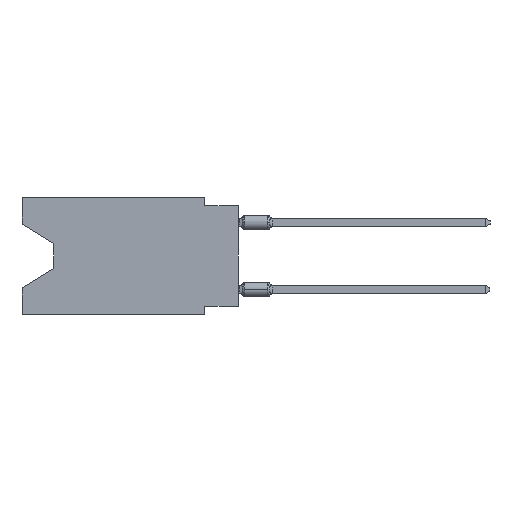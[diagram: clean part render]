
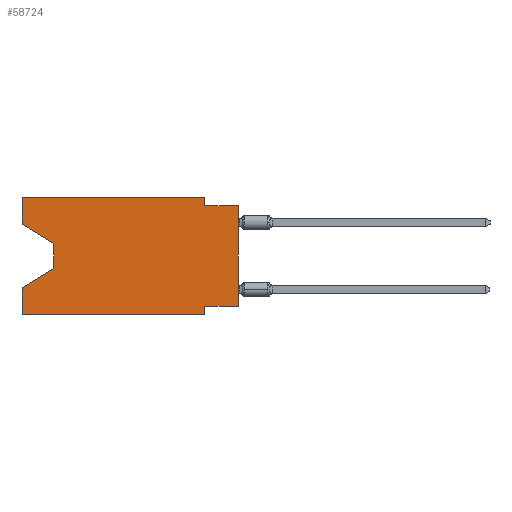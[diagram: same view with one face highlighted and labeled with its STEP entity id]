
A CAD part, left-side view. The second image highlights one B-rep face of the part: STEP entity #58724.
In plain terms, the highlighted planar face has unit normal (-1, 0, 0).
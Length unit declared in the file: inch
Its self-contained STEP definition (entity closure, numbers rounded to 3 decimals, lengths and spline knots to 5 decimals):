
#293 = VERTEX_POINT ( 'NONE', #399 ) ;
#399 = CARTESIAN_POINT ( 'NONE',  ( 0., 0.645, -0.35 ) ) ;
#412 = CARTESIAN_POINT ( 'NONE',  ( 0., 0., -0.325 ) ) ;
#1284 = VERTEX_POINT ( 'NONE', #28639 ) ;
#1549 = DIRECTION ( 'NONE',  ( 0., 0., -1. ) ) ;
#2356 = VECTOR ( 'NONE', #36975, 39.37008 ) ;
#4718 = ORIENTED_EDGE ( 'NONE', *, *, #58949, .F. ) ;
#4814 = VERTEX_POINT ( 'NONE', #9503 ) ;
#4859 = ORIENTED_EDGE ( 'NONE', *, *, #10549, .F. ) ;
#5042 = CARTESIAN_POINT ( 'NONE',  ( 0., 0.1, 0. ) ) ;
#6715 = CARTESIAN_POINT ( 'NONE',  ( 0., 0.645, -0.08025 ) ) ;
#7134 = EDGE_CURVE ( 'NONE', #57390, #23682, #11436, .T. ) ;
#7167 = DIRECTION ( 'NONE',  ( 0., -1., 0. ) ) ;
#7560 = EDGE_CURVE ( 'NONE', #19858, #56398, #16122, .T. ) ;
#7784 = ORIENTED_EDGE ( 'NONE', *, *, #7134, .T. ) ;
#8403 = CARTESIAN_POINT ( 'NONE',  ( 0., 0.645, 0. ) ) ;
#8684 = ORIENTED_EDGE ( 'NONE', *, *, #8702, .T. ) ;
#8702 = EDGE_CURVE ( 'NONE', #293, #1284, #29754, .T. ) ;
#9482 = CARTESIAN_POINT ( 'NONE',  ( 0., 0.645, 0. ) ) ;
#9503 = CARTESIAN_POINT ( 'NONE',  ( 0., 0.645, 0. ) ) ;
#9857 = VERTEX_POINT ( 'NONE', #5042 ) ;
#9894 = EDGE_CURVE ( 'NONE', #4814, #9857, #15497, .T. ) ;
#10064 = VECTOR ( 'NONE', #11071, 39.37008 ) ;
#10549 = EDGE_CURVE ( 'NONE', #57390, #4814, #12846, .T. ) ;
#10797 = CARTESIAN_POINT ( 'NONE',  ( 0., 0.55, -0.212 ) ) ;
#11071 = DIRECTION ( 'NONE',  ( 0., -1., 0. ) ) ;
#11100 = VERTEX_POINT ( 'NONE', #32286 ) ;
#11254 = ORIENTED_EDGE ( 'NONE', *, *, #7560, .T. ) ;
#11359 = DIRECTION ( 'NONE',  ( 0., 0., 1. ) ) ;
#11436 = LINE ( 'NONE', #6715, #28349 ) ;
#11443 = DIRECTION ( 'NONE',  ( 0., 0., -1. ) ) ;
#12846 = LINE ( 'NONE', #8403, #32536 ) ;
#15497 = LINE ( 'NONE', #9482, #42504 ) ;
#15634 = ORIENTED_EDGE ( 'NONE', *, *, #29944, .F. ) ;
#15951 = CARTESIAN_POINT ( 'NONE',  ( 0., 0., -0.025 ) ) ;
#16122 = LINE ( 'NONE', #30372, #46452 ) ;
#16690 = DIRECTION ( 'NONE',  ( 1., 0., 0. ) ) ;
#17109 = DIRECTION ( 'NONE',  ( 0., -0.855, -0.519 ) ) ;
#17300 = FACE_OUTER_BOUND ( 'NONE', #20377, .T. ) ;
#17316 = DIRECTION ( 'NONE',  ( 0., 1., 0. ) ) ;
#17318 = LINE ( 'NONE', #33125, #2356 ) ;
#18092 = ORIENTED_EDGE ( 'NONE', *, *, #35099, .F. ) ;
#18210 = LINE ( 'NONE', #47348, #30458 ) ;
#19685 = LINE ( 'NONE', #39629, #57870 ) ;
#19858 = VERTEX_POINT ( 'NONE', #412 ) ;
#20377 = EDGE_LOOP ( 'NONE', ( #7784, #24432, #31296, #4718, #8684, #18092, #56166, #11254, #15634, #20967, #50102, #4859 ) ) ;
#20805 = PLANE ( 'NONE',  #24362 ) ;
#20967 = ORIENTED_EDGE ( 'NONE', *, *, #57266, .F. ) ;
#22225 = EDGE_CURVE ( 'NONE', #23682, #27014, #17318, .T. ) ;
#22355 = CARTESIAN_POINT ( 'NONE',  ( 0., 0.55, -0.138 ) ) ;
#23670 = EDGE_CURVE ( 'NONE', #19858, #52876, #26193, .T. ) ;
#23682 = VERTEX_POINT ( 'NONE', #22355 ) ;
#24362 = AXIS2_PLACEMENT_3D ( 'NONE', #54686, #16690, #36625 ) ;
#24432 = ORIENTED_EDGE ( 'NONE', *, *, #22225, .T. ) ;
#25853 = LINE ( 'NONE', #29666, #55016 ) ;
#26020 = EDGE_CURVE ( 'NONE', #27014, #11100, #49400, .T. ) ;
#26193 = LINE ( 'NONE', #30968, #47989 ) ;
#27014 = VERTEX_POINT ( 'NONE', #28735 ) ;
#28252 = VECTOR ( 'NONE', #1549, 39.37008 ) ;
#28349 = VECTOR ( 'NONE', #17109, 39.37008 ) ;
#28639 = CARTESIAN_POINT ( 'NONE',  ( 0., 0.1, -0.35 ) ) ;
#28735 = CARTESIAN_POINT ( 'NONE',  ( 0., 0.55, -0.212 ) ) ;
#29103 = DIRECTION ( 'NONE',  ( 0., -1., 0. ) ) ;
#29666 = CARTESIAN_POINT ( 'NONE',  ( 0., 0., -0.025 ) ) ;
#29754 = LINE ( 'NONE', #49070, #10064 ) ;
#29944 = EDGE_CURVE ( 'NONE', #35772, #56398, #25853, .T. ) ;
#30372 = CARTESIAN_POINT ( 'NONE',  ( 0., 0., 0. ) ) ;
#30458 = VECTOR ( 'NONE', #32812, 39.37008 ) ;
#30968 = CARTESIAN_POINT ( 'NONE',  ( 0., 0., -0.325 ) ) ;
#31296 = ORIENTED_EDGE ( 'NONE', *, *, #26020, .T. ) ;
#32286 = CARTESIAN_POINT ( 'NONE',  ( 0., 0.645, -0.26975 ) ) ;
#32536 = VECTOR ( 'NONE', #51151, 39.37008 ) ;
#32812 = DIRECTION ( 'NONE',  ( 0., 0., 1. ) ) ;
#33125 = CARTESIAN_POINT ( 'NONE',  ( 0., 0.55, -0.138 ) ) ;
#35099 = EDGE_CURVE ( 'NONE', #52876, #1284, #19685, .T. ) ;
#35772 = VERTEX_POINT ( 'NONE', #60117 ) ;
#36625 = DIRECTION ( 'NONE',  ( 0., 0., -1. ) ) ;
#36975 = DIRECTION ( 'NONE',  ( 0., 0., -1. ) ) ;
#39629 = CARTESIAN_POINT ( 'NONE',  ( 0., 0.1, -0.35 ) ) ;
#39653 = CARTESIAN_POINT ( 'NONE',  ( 0., 0.1, -0.325 ) ) ;
#42504 = VECTOR ( 'NONE', #29103, 39.37008 ) ;
#44292 = CARTESIAN_POINT ( 'NONE',  ( 0., 0.1, 0. ) ) ;
#46452 = VECTOR ( 'NONE', #11359, 39.37008 ) ;
#47348 = CARTESIAN_POINT ( 'NONE',  ( 0., 0.645, 0. ) ) ;
#47989 = VECTOR ( 'NONE', #17316, 39.37008 ) ;
#48441 = DIRECTION ( 'NONE',  ( 0., 0.855, -0.519 ) ) ;
#49070 = CARTESIAN_POINT ( 'NONE',  ( 0., 0.645, -0.35 ) ) ;
#49400 = LINE ( 'NONE', #10797, #57165 ) ;
#50102 = ORIENTED_EDGE ( 'NONE', *, *, #9894, .F. ) ;
#51151 = DIRECTION ( 'NONE',  ( 0., 0., 1. ) ) ;
#52876 = VERTEX_POINT ( 'NONE', #39653 ) ;
#54686 = CARTESIAN_POINT ( 'NONE',  ( 0., 0.645, 0. ) ) ;
#55016 = VECTOR ( 'NONE', #7167, 39.37008 ) ;
#56166 = ORIENTED_EDGE ( 'NONE', *, *, #23670, .F. ) ;
#56398 = VERTEX_POINT ( 'NONE', #15951 ) ;
#57165 = VECTOR ( 'NONE', #48441, 39.37008 ) ;
#57266 = EDGE_CURVE ( 'NONE', #9857, #35772, #58844, .T. ) ;
#57390 = VERTEX_POINT ( 'NONE', #61363 ) ;
#57870 = VECTOR ( 'NONE', #11443, 39.37008 ) ;
#58724 = ADVANCED_FACE ( 'NONE', ( #17300 ), #20805, .F. ) ;
#58844 = LINE ( 'NONE', #44292, #28252 ) ;
#58949 = EDGE_CURVE ( 'NONE', #293, #11100, #18210, .T. ) ;
#60117 = CARTESIAN_POINT ( 'NONE',  ( 0., 0.1, -0.025 ) ) ;
#61363 = CARTESIAN_POINT ( 'NONE',  ( 0., 0.645, -0.08025 ) ) ;
